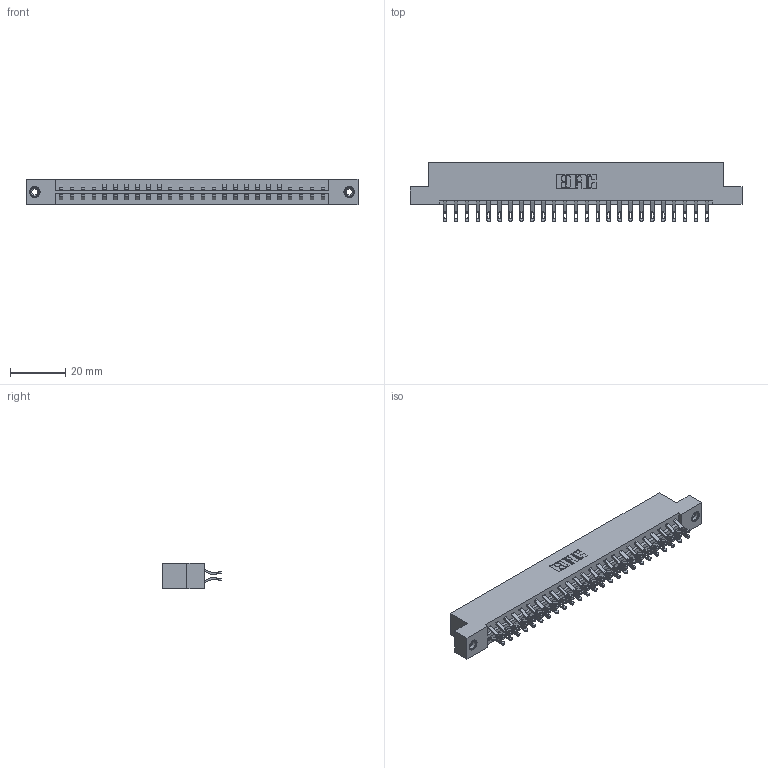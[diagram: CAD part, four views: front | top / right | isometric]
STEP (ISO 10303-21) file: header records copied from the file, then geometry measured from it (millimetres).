
FILE_DESCRIPTION (( 'STEP AP203' ), '1' );
FILE_NAME ('333-050-555-208.STEP', '2018-08-04T01:14:46', ( '' ), ( '' ), 'SwSTEP 2.0', 'SolidWorks 2016', '' );
FILE_SCHEMA (( 'CONFIG_CONTROL_DESIGN' ));
Length unit declared in the file: inch
Products named in the file (4): 333 Part_Flush - .156 Dia - TI; 345-292-001_555 Tail; 345-250-001_345-250-003-102; 333-050-555-208
Assembly tree (53 placements, depth 2):
  333-050-555-208
    333 Part_Flush - .156 Dia - TI
    345-292-001_555 Tail  x50
    345-250-001_345-250-003-102  x2
Bounding box: 120.6 x 21.47 x 9.4 mm (x, y, z)
Volume: 12292 mm3; surface area: 14913.7 mm2
Topology: 53 solids, 53 shells, 3074 faces, 9597 edges, 6390 vertices
Faces by surface type: plane 1802, cylinder 1256, cone 12, torus 4
Entity records: 19794 total; most frequent: CARTESIAN_POINT 3319, ORIENTED_EDGE 3218, DIRECTION 2867, EDGE_CURVE 1609, VECTOR 1441, LINE 1441, VERTEX_POINT 1068, AXIS2_PLACEMENT_3D 713
